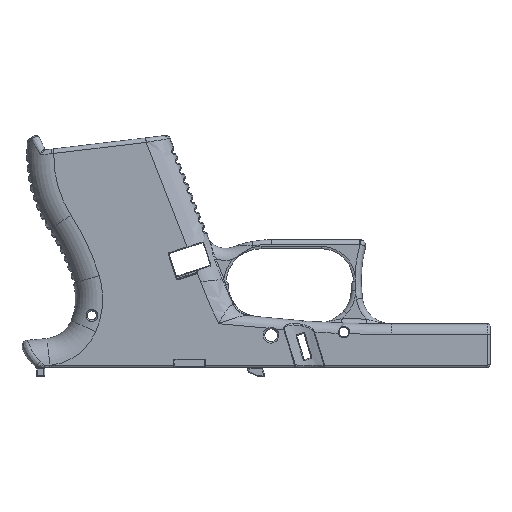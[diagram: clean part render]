
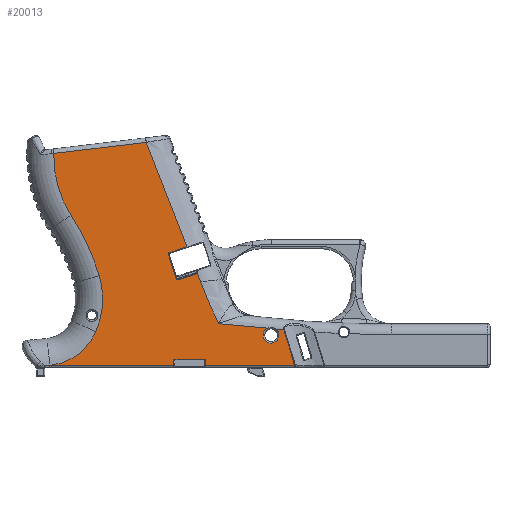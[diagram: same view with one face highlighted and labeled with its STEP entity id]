
A CAD part, front view. The second image highlights one B-rep face of the part: STEP entity #20013.
In plain terms, the highlighted planar face has unit normal (0, -1, 0).
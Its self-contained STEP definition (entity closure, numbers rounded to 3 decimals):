
#173=PLANE('',#21535);
#758=LINE('',#33217,#1808);
#759=LINE('',#33219,#1809);
#760=LINE('',#33253,#1810);
#768=LINE('',#33306,#1818);
#769=LINE('',#33313,#1819);
#770=LINE('',#33315,#1820);
#771=LINE('',#33317,#1821);
#772=LINE('',#33319,#1822);
#773=LINE('',#33325,#1823);
#774=LINE('',#33329,#1824);
#775=LINE('',#33333,#1825);
#776=LINE('',#33337,#1826);
#777=LINE('',#33341,#1827);
#778=LINE('',#33343,#1828);
#779=LINE('',#33345,#1829);
#780=LINE('',#33352,#1830);
#781=LINE('',#33353,#1831);
#1808=VECTOR('',#24505,10.);
#1809=VECTOR('',#24508,10.);
#1810=VECTOR('',#24513,10.);
#1818=VECTOR('',#24541,10.);
#1819=VECTOR('',#24552,10.);
#1820=VECTOR('',#24553,10.);
#1821=VECTOR('',#24554,10.);
#1822=VECTOR('',#24555,10.);
#1823=VECTOR('',#24560,10.);
#1824=VECTOR('',#24563,10.);
#1825=VECTOR('',#24566,10.);
#1826=VECTOR('',#24569,10.);
#1827=VECTOR('',#24572,10.);
#1828=VECTOR('',#24573,10.);
#1829=VECTOR('',#24574,10.);
#1830=VECTOR('',#24581,10.);
#1831=VECTOR('',#24582,10.);
#3767=FACE_OUTER_BOUND('',#5087,.T.);
#5087=EDGE_LOOP('',(#13941,#13942,#13943,#13944,#13945,#13946,#13947,#13948,
#13949,#13950,#13951,#13952,#13953,#13954,#13955,#13956,#13957,#13958,#13959,
#13960,#13961,#13962,#13963,#13964,#13965,#13966,#13967,#13968));
#6603=CIRCLE('',#21264,27.167);
#6737=CIRCLE('',#21523,0.8);
#6742=CIRCLE('',#21536,2.625);
#6743=CIRCLE('',#21537,2.625);
#6744=CIRCLE('',#21538,156.771);
#6745=CIRCLE('',#21539,0.49);
#6746=CIRCLE('',#21540,0.49);
#6747=CIRCLE('',#21541,0.49);
#6748=CIRCLE('',#21542,35.645);
#6749=CIRCLE('',#21543,77.599);
#6750=CIRCLE('',#21544,18.891);
#7905=VERTEX_POINT('',#30270);
#7906=VERTEX_POINT('',#30272);
#8244=VERTEX_POINT('',#32868);
#8266=VERTEX_POINT('',#33037);
#8282=VERTEX_POINT('',#33215);
#8283=VERTEX_POINT('',#33244);
#8285=VERTEX_POINT('',#33282);
#8293=VERTEX_POINT('',#33304);
#8294=VERTEX_POINT('',#33312);
#8295=VERTEX_POINT('',#33314);
#8296=VERTEX_POINT('',#33316);
#8297=VERTEX_POINT('',#33318);
#8298=VERTEX_POINT('',#33320);
#8299=VERTEX_POINT('',#33322);
#8300=VERTEX_POINT('',#33324);
#8301=VERTEX_POINT('',#33326);
#8302=VERTEX_POINT('',#33328);
#8303=VERTEX_POINT('',#33330);
#8304=VERTEX_POINT('',#33332);
#8305=VERTEX_POINT('',#33334);
#8306=VERTEX_POINT('',#33336);
#8307=VERTEX_POINT('',#33338);
#8308=VERTEX_POINT('',#33340);
#8309=VERTEX_POINT('',#33342);
#8310=VERTEX_POINT('',#33344);
#8311=VERTEX_POINT('',#33346);
#8312=VERTEX_POINT('',#33349);
#8313=VERTEX_POINT('',#33351);
#9854=EDGE_CURVE('',#7905,#7906,#6603,.T.);
#10347=EDGE_CURVE('',#8282,#8244,#758,.T.);
#10348=EDGE_CURVE('',#8244,#8266,#759,.T.);
#10351=EDGE_CURVE('',#8266,#8283,#760,.T.);
#10354=EDGE_CURVE('',#8283,#8285,#6737,.T.);
#10366=EDGE_CURVE('',#8293,#8282,#768,.T.);
#10369=EDGE_CURVE('',#8294,#8293,#769,.T.);
#10370=EDGE_CURVE('',#8295,#8294,#770,.T.);
#10371=EDGE_CURVE('',#8296,#8295,#771,.T.);
#10372=EDGE_CURVE('',#8297,#8296,#772,.T.);
#10373=EDGE_CURVE('',#8298,#8297,#6742,.T.);
#10374=EDGE_CURVE('',#8299,#8298,#6743,.T.);
#10375=EDGE_CURVE('',#8300,#8299,#773,.T.);
#10376=EDGE_CURVE('',#8301,#8300,#6744,.T.);
#10377=EDGE_CURVE('',#8301,#8302,#774,.T.);
#10378=EDGE_CURVE('',#8303,#8302,#6745,.T.);
#10379=EDGE_CURVE('',#8304,#8303,#775,.T.);
#10380=EDGE_CURVE('',#8305,#8304,#6746,.T.);
#10381=EDGE_CURVE('',#8306,#8305,#776,.T.);
#10382=EDGE_CURVE('',#8307,#8306,#6747,.T.);
#10383=EDGE_CURVE('',#8308,#8307,#777,.T.);
#10384=EDGE_CURVE('',#8308,#8309,#778,.T.);
#10385=EDGE_CURVE('',#8310,#8309,#779,.T.);
#10386=EDGE_CURVE('',#8311,#8310,#6748,.T.);
#10387=EDGE_CURVE('',#7906,#8311,#6749,.T.);
#10388=EDGE_CURVE('',#8312,#7905,#6750,.T.);
#10389=EDGE_CURVE('',#8313,#8312,#780,.T.);
#10390=EDGE_CURVE('',#8285,#8313,#781,.T.);
#13941=ORIENTED_EDGE('',*,*,#10347,.F.);
#13942=ORIENTED_EDGE('',*,*,#10366,.F.);
#13943=ORIENTED_EDGE('',*,*,#10369,.F.);
#13944=ORIENTED_EDGE('',*,*,#10370,.F.);
#13945=ORIENTED_EDGE('',*,*,#10371,.F.);
#13946=ORIENTED_EDGE('',*,*,#10372,.F.);
#13947=ORIENTED_EDGE('',*,*,#10373,.F.);
#13948=ORIENTED_EDGE('',*,*,#10374,.F.);
#13949=ORIENTED_EDGE('',*,*,#10375,.F.);
#13950=ORIENTED_EDGE('',*,*,#10376,.F.);
#13951=ORIENTED_EDGE('',*,*,#10377,.T.);
#13952=ORIENTED_EDGE('',*,*,#10378,.F.);
#13953=ORIENTED_EDGE('',*,*,#10379,.F.);
#13954=ORIENTED_EDGE('',*,*,#10380,.F.);
#13955=ORIENTED_EDGE('',*,*,#10381,.F.);
#13956=ORIENTED_EDGE('',*,*,#10382,.F.);
#13957=ORIENTED_EDGE('',*,*,#10383,.F.);
#13958=ORIENTED_EDGE('',*,*,#10384,.T.);
#13959=ORIENTED_EDGE('',*,*,#10385,.F.);
#13960=ORIENTED_EDGE('',*,*,#10386,.F.);
#13961=ORIENTED_EDGE('',*,*,#10387,.F.);
#13962=ORIENTED_EDGE('',*,*,#9854,.F.);
#13963=ORIENTED_EDGE('',*,*,#10388,.F.);
#13964=ORIENTED_EDGE('',*,*,#10389,.F.);
#13965=ORIENTED_EDGE('',*,*,#10390,.F.);
#13966=ORIENTED_EDGE('',*,*,#10354,.F.);
#13967=ORIENTED_EDGE('',*,*,#10351,.F.);
#13968=ORIENTED_EDGE('',*,*,#10348,.F.);
#20013=ADVANCED_FACE('',(#3767),#173,.F.);
#21264=AXIS2_PLACEMENT_3D('',#30273,#23783,#23784);
#21523=AXIS2_PLACEMENT_3D('',#33283,#24518,#24519);
#21535=AXIS2_PLACEMENT_3D('',#33311,#24550,#24551);
#21536=AXIS2_PLACEMENT_3D('',#33321,#24556,#24557);
#21537=AXIS2_PLACEMENT_3D('',#33323,#24558,#24559);
#21538=AXIS2_PLACEMENT_3D('',#33327,#24561,#24562);
#21539=AXIS2_PLACEMENT_3D('',#33331,#24564,#24565);
#21540=AXIS2_PLACEMENT_3D('',#33335,#24567,#24568);
#21541=AXIS2_PLACEMENT_3D('',#33339,#24570,#24571);
#21542=AXIS2_PLACEMENT_3D('',#33347,#24575,#24576);
#21543=AXIS2_PLACEMENT_3D('',#33348,#24577,#24578);
#21544=AXIS2_PLACEMENT_3D('',#33350,#24579,#24580);
#23783=DIRECTION('center_axis',(0.,-1.,0.));
#23784=DIRECTION('ref_axis',(0.998,0.,-0.06));
#24505=DIRECTION('',(0.,0.,1.));
#24508=DIRECTION('',(-1.,0.,0.));
#24513=DIRECTION('',(0.,0.,-1.));
#24518=DIRECTION('center_axis',(0.,-1.,0.));
#24519=DIRECTION('ref_axis',(-0.707,0.,0.707));
#24541=DIRECTION('',(-1.,0.,0.));
#24550=DIRECTION('center_axis',(0.,1.,0.));
#24551=DIRECTION('ref_axis',(1.,0.,0.));
#24552=DIRECTION('',(0.,0.,1.));
#24553=DIRECTION('',(-1.,0.,0.));
#24554=DIRECTION('',(0.292,0.,-0.956));
#24555=DIRECTION('',(0.996,0.,-0.092));
#24556=DIRECTION('center_axis',(0.,-1.,0.));
#24557=DIRECTION('ref_axis',(-1.,0.,0.));
#24558=DIRECTION('center_axis',(0.,-1.,0.));
#24559=DIRECTION('ref_axis',(-1.,0.,0.));
#24560=DIRECTION('',(0.996,0.,-0.092));
#24561=DIRECTION('center_axis',(0.,-1.,0.));
#24562=DIRECTION('ref_axis',(-0.937,0.,-0.35));
#24563=DIRECTION('',(-0.363,0.,0.932));
#24564=DIRECTION('center_axis',(0.,-1.,0.));
#24565=DIRECTION('ref_axis',(0.891,0.,-0.454));
#24566=DIRECTION('',(0.951,0.,0.309));
#24567=DIRECTION('center_axis',(0.,-1.,0.));
#24568=DIRECTION('ref_axis',(-0.454,0.,-0.891));
#24569=DIRECTION('',(0.309,0.,-0.951));
#24570=DIRECTION('center_axis',(0.,-1.,0.));
#24571=DIRECTION('ref_axis',(-0.891,0.,0.454));
#24572=DIRECTION('',(-0.951,0.,-0.309));
#24573=DIRECTION('',(-0.363,0.,0.932));
#24574=DIRECTION('',(0.993,0.,0.119));
#24575=DIRECTION('center_axis',(0.,1.,0.));
#24576=DIRECTION('ref_axis',(-0.961,0.,-0.276));
#24577=DIRECTION('center_axis',(0.,-1.,0.));
#24578=DIRECTION('ref_axis',(0.907,0.,0.421));
#24579=DIRECTION('center_axis',(0.,-1.,0.));
#24580=DIRECTION('ref_axis',(0.592,0.,-0.806));
#24581=DIRECTION('',(-1.,0.,0.));
#24582=DIRECTION('',(0.,0.,-1.));
#30270=CARTESIAN_POINT('',(-55.002,-11.5,-14.602));
#30272=CARTESIAN_POINT('',(-53.881,-11.5,4.09));
#30273=CARTESIAN_POINT('Origin',(-79.899,-11.5,-3.729));
#32868=CARTESIAN_POINT('',(-18.52,-11.5,-23.745));
#33037=CARTESIAN_POINT('',(-28.98,-11.5,-23.745));
#33215=CARTESIAN_POINT('',(-18.52,-11.5,-24.675));
#33217=CARTESIAN_POINT('',(-18.52,-11.5,-7.056));
#33219=CARTESIAN_POINT('',(-10.264,-11.5,-23.745));
#33244=CARTESIAN_POINT('',(-28.98,-11.5,-25.148));
#33253=CARTESIAN_POINT('',(-28.98,-11.5,-7.056));
#33282=CARTESIAN_POINT('',(-29.05,-11.5,-25.475));
#33283=CARTESIAN_POINT('Origin',(-28.25,-11.5,-25.475));
#33304=CARTESIAN_POINT('',(-18.45,-11.5,-24.675));
#33306=CARTESIAN_POINT('',(-10.264,-11.5,-24.675));
#33311=CARTESIAN_POINT('Origin',(-1.777,-11.5,10.863));
#33312=CARTESIAN_POINT('',(-18.45,-11.5,-25.75));
#33313=CARTESIAN_POINT('',(-18.45,-11.5,-7.818));
#33314=CARTESIAN_POINT('',(11.185,-11.5,-25.75));
#33315=CARTESIAN_POINT('',(37.236,-11.5,-25.75));
#33316=CARTESIAN_POINT('',(7.57,-11.5,-13.924));
#33317=CARTESIAN_POINT('',(5.553,-11.5,-7.328));
#33318=CARTESIAN_POINT('',(4.906,-11.5,-13.679));
#33319=CARTESIAN_POINT('',(4.861,-11.5,-13.675));
#33320=CARTESIAN_POINT('',(5.968,-11.5,-15.788));
#33321=CARTESIAN_POINT('Origin',(3.343,-11.5,-15.788));
#33322=CARTESIAN_POINT('',(2.19,-11.5,-13.43));
#33323=CARTESIAN_POINT('Origin',(3.343,-11.5,-15.788));
#33324=CARTESIAN_POINT('',(-14.141,-11.5,-11.929));
#33325=CARTESIAN_POINT('',(4.861,-11.5,-13.675));
#33326=CARTESIAN_POINT('',(-20.166,-11.5,2.06));
#33327=CARTESIAN_POINT('Origin',(126.663,-11.5,57.001));
#33328=CARTESIAN_POINT('',(-21.238,-11.5,4.813));
#33329=CARTESIAN_POINT('',(-37.545,-11.5,46.678));
#33330=CARTESIAN_POINT('',(-21.428,-11.5,4.698));
#33331=CARTESIAN_POINT('Origin',(-21.58,-11.5,5.164));
#33332=CARTESIAN_POINT('',(-27.61,-11.5,2.69));
#33333=CARTESIAN_POINT('',(-11.516,-11.5,7.919));
#33334=CARTESIAN_POINT('',(-28.228,-11.5,3.004));
#33335=CARTESIAN_POINT('Origin',(-27.762,-11.5,3.156));
#33336=CARTESIAN_POINT('',(-30.854,-11.5,11.088));
#33337=CARTESIAN_POINT('',(-28.236,-11.5,3.028));
#33338=CARTESIAN_POINT('',(-30.54,-11.5,11.706));
#33339=CARTESIAN_POINT('Origin',(-30.388,-11.5,11.24));
#33340=CARTESIAN_POINT('',(-24.666,-11.5,13.614));
#33341=CARTESIAN_POINT('',(-17.775,-11.5,15.853));
#33342=CARTESIAN_POINT('',(-38.228,-11.5,48.431));
#33343=CARTESIAN_POINT('',(-37.545,-11.5,46.678));
#33344=CARTESIAN_POINT('',(-68.991,-11.5,44.75));
#33345=CARTESIAN_POINT('',(-18.413,-11.5,50.802));
#33346=CARTESIAN_POINT('',(-63.213,-11.5,24.169));
#33347=CARTESIAN_POINT('Origin',(-33.363,-11.5,43.651));
#33348=CARTESIAN_POINT('Origin',(-128.196,-11.5,-18.243));
#33349=CARTESIAN_POINT('',(-69.695,-11.5,-25.75));
#33350=CARTESIAN_POINT('Origin',(-72.315,-11.5,-7.041));
#33351=CARTESIAN_POINT('',(-29.05,-11.5,-25.75));
#33352=CARTESIAN_POINT('',(37.236,-11.5,-25.75));
#33353=CARTESIAN_POINT('',(-29.05,-11.5,-7.056));
